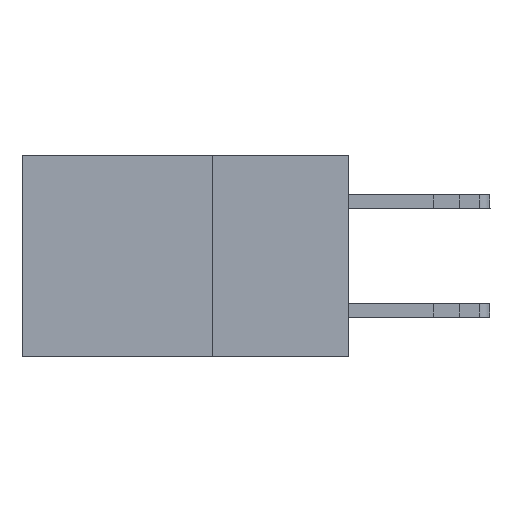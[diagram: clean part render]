
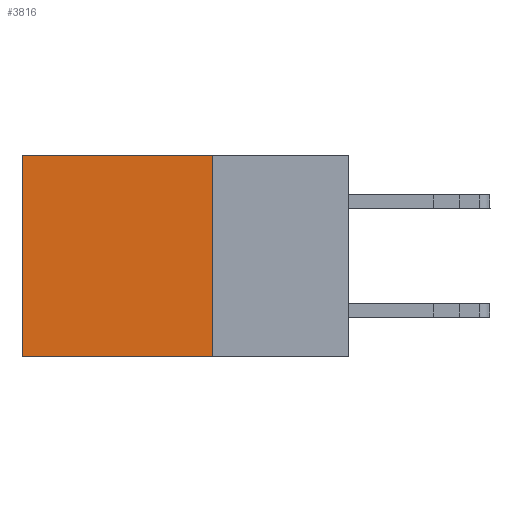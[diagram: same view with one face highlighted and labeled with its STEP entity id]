
A CAD part, left-side view. The second image highlights one B-rep face of the part: STEP entity #3816.
In plain terms, the highlighted planar face has unit normal (-1, 0, 0).
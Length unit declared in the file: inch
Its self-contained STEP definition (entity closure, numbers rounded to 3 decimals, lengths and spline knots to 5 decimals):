
#766 = LINE ( 'NONE', #10552, #3584 ) ;
#1142 = PLANE ( 'NONE',  #10459 ) ;
#1471 = EDGE_CURVE ( 'NONE', #8553, #8776, #766, .T. ) ;
#1665 = VECTOR ( 'NONE', #15928, 39.37008 ) ;
#2978 = DIRECTION ( 'NONE',  ( 0., 0., -1. ) ) ;
#3255 = VERTEX_POINT ( 'NONE', #13916 ) ;
#3367 = EDGE_CURVE ( 'NONE', #13951, #3255, #15818, .T. ) ;
#3584 = VECTOR ( 'NONE', #15568, 39.37008 ) ;
#3816 = ADVANCED_FACE ( 'NONE', ( #7305 ), #1142, .F. ) ;
#4691 = DIRECTION ( 'NONE',  ( 0., 1., 0. ) ) ;
#5477 = ORIENTED_EDGE ( 'NONE', *, *, #3367, .F. ) ;
#6055 = CARTESIAN_POINT ( 'NONE',  ( 0.2615, 0.25, -0.37 ) ) ;
#6237 = CARTESIAN_POINT ( 'NONE',  ( 0.2615, 0.25, -0.37 ) ) ;
#7065 = VECTOR ( 'NONE', #4691, 39.37008 ) ;
#7171 = CARTESIAN_POINT ( 'NONE',  ( 0.2615, 0.25, -0.37 ) ) ;
#7305 = FACE_OUTER_BOUND ( 'NONE', #15154, .T. ) ;
#7438 = ORIENTED_EDGE ( 'NONE', *, *, #1471, .T. ) ;
#7796 = EDGE_CURVE ( 'NONE', #8553, #13951, #13377, .T. ) ;
#8547 = ORIENTED_EDGE ( 'NONE', *, *, #7796, .F. ) ;
#8553 = VERTEX_POINT ( 'NONE', #10544 ) ;
#8776 = VERTEX_POINT ( 'NONE', #11423 ) ;
#9095 = LINE ( 'NONE', #11697, #15742 ) ;
#10459 = AXIS2_PLACEMENT_3D ( 'NONE', #6237, #12481, #15020 ) ;
#10538 = EDGE_CURVE ( 'NONE', #8776, #3255, #9095, .T. ) ;
#10544 = CARTESIAN_POINT ( 'NONE',  ( 0.2615, 0.25, 0. ) ) ;
#10552 = CARTESIAN_POINT ( 'NONE',  ( 0.2615, 0.25, 0. ) ) ;
#10841 = CARTESIAN_POINT ( 'NONE',  ( 0.2615, 0.25, -0.37 ) ) ;
#11423 = CARTESIAN_POINT ( 'NONE',  ( 0.2615, 0.6, 0. ) ) ;
#11697 = CARTESIAN_POINT ( 'NONE',  ( 0.2615, 0.6, -0.37 ) ) ;
#12481 = DIRECTION ( 'NONE',  ( 1., 0., 0. ) ) ;
#13377 = LINE ( 'NONE', #6055, #1665 ) ;
#13916 = CARTESIAN_POINT ( 'NONE',  ( 0.2615, 0.6, -0.37 ) ) ;
#13951 = VERTEX_POINT ( 'NONE', #10841 ) ;
#14004 = ORIENTED_EDGE ( 'NONE', *, *, #10538, .T. ) ;
#15020 = DIRECTION ( 'NONE',  ( 0., 0., -1. ) ) ;
#15154 = EDGE_LOOP ( 'NONE', ( #14004, #5477, #8547, #7438 ) ) ;
#15568 = DIRECTION ( 'NONE',  ( 0., 1., 0. ) ) ;
#15742 = VECTOR ( 'NONE', #2978, 39.37008 ) ;
#15818 = LINE ( 'NONE', #7171, #7065 ) ;
#15928 = DIRECTION ( 'NONE',  ( 0., 0., -1. ) ) ;
